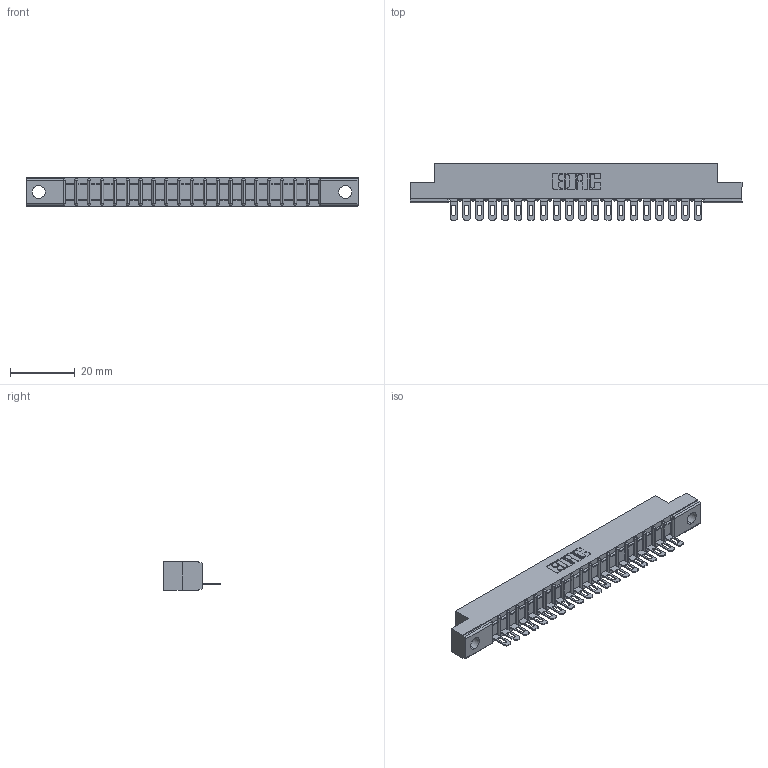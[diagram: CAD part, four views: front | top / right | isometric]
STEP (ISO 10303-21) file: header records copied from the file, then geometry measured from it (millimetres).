
FILE_DESCRIPTION (( 'STEP AP203' ), '1' );
FILE_NAME ('357-020-501-104.STEP', '2018-08-08T07:52:14', ( '' ), ( '' ), 'SwSTEP 2.0', 'SolidWorks 2016', '' );
FILE_SCHEMA (( 'CONFIG_CONTROL_DESIGN' ));
Length unit declared in the file: inch
Products named in the file (3): 307 Part_.156 Dia Mounting Holes; 307-290-002_501; 357-020-501-104
Assembly tree (21 placements, depth 2):
  357-020-501-104
    307 Part_.156 Dia Mounting Holes
    307-290-002_501  x20
Bounding box: 102.26 x 17.42 x 8.71 mm (x, y, z)
Volume: 6661.5 mm3; surface area: 12030.2 mm2
Topology: 21 solids, 21 shells, 1673 faces, 5119 edges, 3354 vertices
Faces by surface type: plane 964, cylinder 667, sphere 42
Entity records: 21070 total; most frequent: CARTESIAN_POINT 3554, ORIENTED_EDGE 3542, DIRECTION 3459, EDGE_CURVE 1771, LINE 1349, VECTOR 1349, VERTEX_POINT 1150, AXIS2_PLACEMENT_3D 1055
